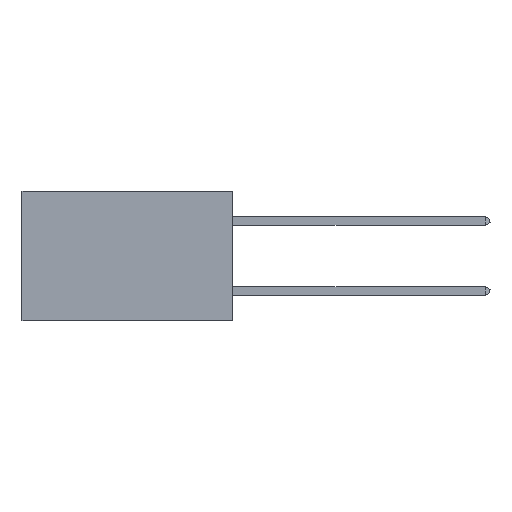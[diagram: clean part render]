
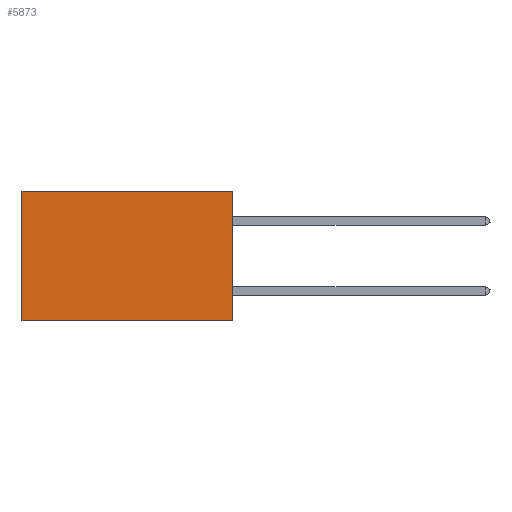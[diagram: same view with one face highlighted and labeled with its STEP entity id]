
A CAD part, left-side view. The second image highlights one B-rep face of the part: STEP entity #5873.
In plain terms, the highlighted planar face has unit normal (-1, 0, 0).
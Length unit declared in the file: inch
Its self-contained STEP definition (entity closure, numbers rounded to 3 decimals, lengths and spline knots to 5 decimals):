
#10 = CARTESIAN_POINT ( 'NONE',  ( 0.2875, 0., 0. ) ) ;
#800 = VECTOR ( 'NONE', #33598, 39.37008 ) ;
#1645 = ORIENTED_EDGE ( 'NONE', *, *, #2938, .F. ) ;
#1800 = VERTEX_POINT ( 'NONE', #22871 ) ;
#1900 = CARTESIAN_POINT ( 'NONE',  ( 0.2875, 0., 0. ) ) ;
#2402 = DIRECTION ( 'NONE',  ( 1., 0., 0. ) ) ;
#2938 = EDGE_CURVE ( 'NONE', #7957, #1800, #25577, .T. ) ;
#5443 = PLANE ( 'NONE',  #34402 ) ;
#5873 = ADVANCED_FACE ( 'NONE', ( #12504 ), #5443, .F. ) ;
#7844 = DIRECTION ( 'NONE',  ( 0., 0., -1. ) ) ;
#7957 = VERTEX_POINT ( 'NONE', #19235 ) ;
#8770 = VECTOR ( 'NONE', #31539, 39.37008 ) ;
#10902 = LINE ( 'NONE', #35508, #28196 ) ;
#11054 = VERTEX_POINT ( 'NONE', #17669 ) ;
#11066 = LINE ( 'NONE', #1900, #29602 ) ;
#11485 = CARTESIAN_POINT ( 'NONE',  ( 0.2875, 0., 0. ) ) ;
#11759 = CARTESIAN_POINT ( 'NONE',  ( 0.2875, 0., -0.37 ) ) ;
#12504 = FACE_OUTER_BOUND ( 'NONE', #26098, .T. ) ;
#13428 = EDGE_CURVE ( 'NONE', #11054, #1800, #10902, .T. ) ;
#13444 = DIRECTION ( 'NONE',  ( 0., 0., -1. ) ) ;
#15985 = VERTEX_POINT ( 'NONE', #28643 ) ;
#17669 = CARTESIAN_POINT ( 'NONE',  ( 0.2875, 0.6, 0. ) ) ;
#19235 = CARTESIAN_POINT ( 'NONE',  ( 0.2875, 0., -0.37 ) ) ;
#21104 = EDGE_CURVE ( 'NONE', #15985, #11054, #26328, .T. ) ;
#22871 = CARTESIAN_POINT ( 'NONE',  ( 0.2875, 0.6, -0.37 ) ) ;
#22982 = ORIENTED_EDGE ( 'NONE', *, *, #34502, .F. ) ;
#25577 = LINE ( 'NONE', #11759, #8770 ) ;
#26098 = EDGE_LOOP ( 'NONE', ( #32614, #1645, #22982, #35543 ) ) ;
#26328 = LINE ( 'NONE', #11485, #800 ) ;
#27797 = DIRECTION ( 'NONE',  ( 0., 0., -1. ) ) ;
#28196 = VECTOR ( 'NONE', #27797, 39.37008 ) ;
#28643 = CARTESIAN_POINT ( 'NONE',  ( 0.2875, 0., 0. ) ) ;
#29602 = VECTOR ( 'NONE', #7844, 39.37008 ) ;
#31539 = DIRECTION ( 'NONE',  ( 0., 1., 0. ) ) ;
#32614 = ORIENTED_EDGE ( 'NONE', *, *, #13428, .T. ) ;
#33598 = DIRECTION ( 'NONE',  ( 0., 1., 0. ) ) ;
#34402 = AXIS2_PLACEMENT_3D ( 'NONE', #10, #2402, #13444 ) ;
#34502 = EDGE_CURVE ( 'NONE', #15985, #7957, #11066, .T. ) ;
#35508 = CARTESIAN_POINT ( 'NONE',  ( 0.2875, 0.6, 0. ) ) ;
#35543 = ORIENTED_EDGE ( 'NONE', *, *, #21104, .T. ) ;
